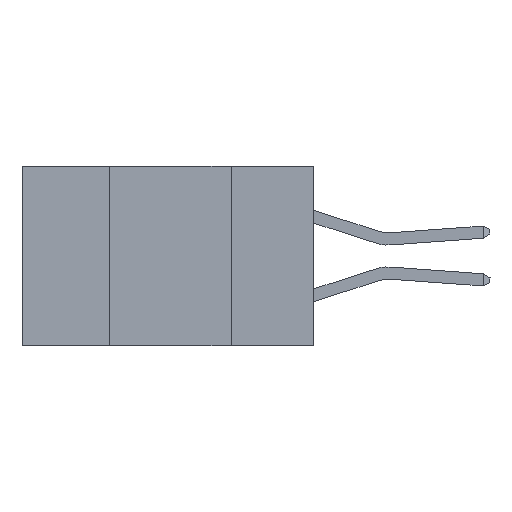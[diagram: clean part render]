
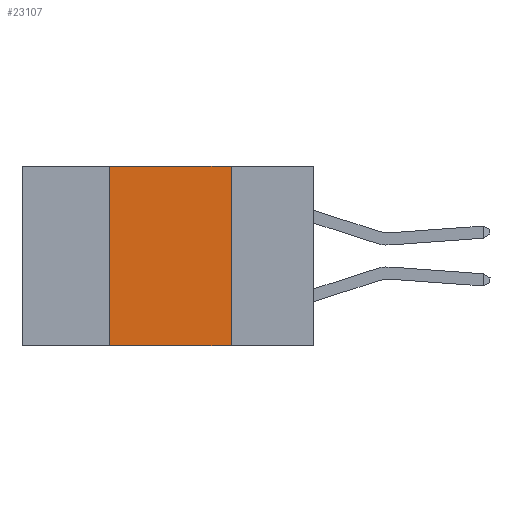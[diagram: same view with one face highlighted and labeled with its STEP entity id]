
A CAD part, left-side view. The second image highlights one B-rep face of the part: STEP entity #23107.
In plain terms, the highlighted planar face has unit normal (-1, 0, 0).
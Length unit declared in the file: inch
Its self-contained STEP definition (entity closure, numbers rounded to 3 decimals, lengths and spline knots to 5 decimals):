
#255 = VECTOR ( 'NONE', #2125, 39.37008 ) ;
#697 = PLANE ( 'NONE',  #17882 ) ;
#1058 = VERTEX_POINT ( 'NONE', #16260 ) ;
#2125 = DIRECTION ( 'NONE',  ( 0., -1., 0. ) ) ;
#2634 = VECTOR ( 'NONE', #16119, 39.37008 ) ;
#2637 = VERTEX_POINT ( 'NONE', #7827 ) ;
#3833 = VERTEX_POINT ( 'NONE', #24264 ) ;
#4126 = DIRECTION ( 'NONE',  ( 0., 0., 1. ) ) ;
#4144 = CARTESIAN_POINT ( 'NONE',  ( 0., 0.6, -0.37 ) ) ;
#7827 = CARTESIAN_POINT ( 'NONE',  ( 0., 0.17, -0.37 ) ) ;
#8215 = EDGE_CURVE ( 'NONE', #1058, #2637, #22324, .T. ) ;
#8714 = VECTOR ( 'NONE', #4126, 39.37008 ) ;
#10296 = CARTESIAN_POINT ( 'NONE',  ( 0., 0.42, 0. ) ) ;
#10606 = EDGE_CURVE ( 'NONE', #13727, #3833, #23383, .T. ) ;
#11285 = FACE_OUTER_BOUND ( 'NONE', #15706, .T. ) ;
#11582 = DIRECTION ( 'NONE',  ( 0., 0., -1. ) ) ;
#11761 = CARTESIAN_POINT ( 'NONE',  ( 0., 0.6, 0. ) ) ;
#12340 = ORIENTED_EDGE ( 'NONE', *, *, #15188, .F. ) ;
#13727 = VERTEX_POINT ( 'NONE', #10296 ) ;
#14107 = CARTESIAN_POINT ( 'NONE',  ( 0., 0.42, 0. ) ) ;
#14442 = CARTESIAN_POINT ( 'NONE',  ( 0., 0.17, 0. ) ) ;
#15188 = EDGE_CURVE ( 'NONE', #3833, #2637, #16164, .T. ) ;
#15250 = ORIENTED_EDGE ( 'NONE', *, *, #8215, .T. ) ;
#15706 = EDGE_LOOP ( 'NONE', ( #12340, #16167, #17514, #15250 ) ) ;
#16117 = DIRECTION ( 'NONE',  ( 0., 0., -1. ) ) ;
#16119 = DIRECTION ( 'NONE',  ( 0., -1., 0. ) ) ;
#16164 = LINE ( 'NONE', #14442, #24630 ) ;
#16167 = ORIENTED_EDGE ( 'NONE', *, *, #10606, .F. ) ;
#16260 = CARTESIAN_POINT ( 'NONE',  ( 0., 0.42, -0.37 ) ) ;
#17514 = ORIENTED_EDGE ( 'NONE', *, *, #19936, .F. ) ;
#17882 = AXIS2_PLACEMENT_3D ( 'NONE', #11761, #23611, #11582 ) ;
#18039 = CARTESIAN_POINT ( 'NONE',  ( 0., 0.6, 0. ) ) ;
#19936 = EDGE_CURVE ( 'NONE', #1058, #13727, #23438, .T. ) ;
#22324 = LINE ( 'NONE', #4144, #255 ) ;
#23107 = ADVANCED_FACE ( 'NONE', ( #11285 ), #697, .F. ) ;
#23383 = LINE ( 'NONE', #18039, #2634 ) ;
#23438 = LINE ( 'NONE', #14107, #8714 ) ;
#23611 = DIRECTION ( 'NONE',  ( 1., 0., 0. ) ) ;
#24264 = CARTESIAN_POINT ( 'NONE',  ( 0., 0.17, 0. ) ) ;
#24630 = VECTOR ( 'NONE', #16117, 39.37008 ) ;
